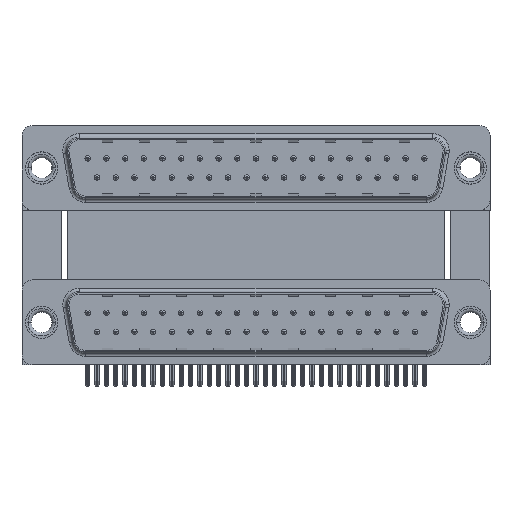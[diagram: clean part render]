
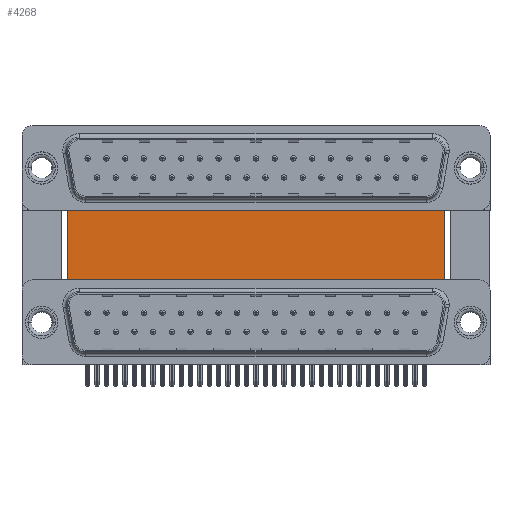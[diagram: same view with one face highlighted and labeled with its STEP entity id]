
A CAD part, top view. The second image highlights one B-rep face of the part: STEP entity #4268.
In plain terms, the highlighted planar face has unit normal (0, 0, 1).
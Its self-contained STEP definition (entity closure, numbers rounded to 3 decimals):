
#3031 = ORIENTED_EDGE ( 'NONE', *, *, #50765, .F. ) ;
#3351 = VECTOR ( 'NONE', #49245, 1000. ) ;
#4268 = ADVANCED_FACE ( 'NONE', ( #32159 ), #43980, .F. ) ;
#5175 = CARTESIAN_POINT ( 'NONE',  ( 3.79, 16.585, -12. ) ) ;
#9388 = CARTESIAN_POINT ( 'NONE',  ( 3.79, 16.585, -12. ) ) ;
#11183 = VECTOR ( 'NONE', #44764, 1000. ) ;
#13521 = CARTESIAN_POINT ( 'NONE',  ( 3.79, 16.585, -12. ) ) ;
#15374 = CARTESIAN_POINT ( 'NONE',  ( 59.71, -3.735, -12. ) ) ;
#17999 = VECTOR ( 'NONE', #21166, 1000. ) ;
#18813 = CARTESIAN_POINT ( 'NONE',  ( 59.71, 16.585, -12. ) ) ;
#19099 = VERTEX_POINT ( 'NONE', #15374 ) ;
#21166 = DIRECTION ( 'NONE',  ( 1., 0., 0. ) ) ;
#21532 = ORIENTED_EDGE ( 'NONE', *, *, #44427, .T. ) ;
#21940 = ORIENTED_EDGE ( 'NONE', *, *, #35504, .F. ) ;
#22211 = DIRECTION ( 'NONE',  ( 0., -1., 0. ) ) ;
#23934 = DIRECTION ( 'NONE',  ( 0., 0., -1. ) ) ;
#24720 = LINE ( 'NONE', #5175, #11183 ) ;
#26570 = LINE ( 'NONE', #42001, #46527 ) ;
#28113 = CARTESIAN_POINT ( 'NONE',  ( 3.79, -3.735, -12. ) ) ;
#28541 = DIRECTION ( 'NONE',  ( -1., 0., 0. ) ) ;
#32159 = FACE_OUTER_BOUND ( 'NONE', #48463, .T. ) ;
#32413 = CARTESIAN_POINT ( 'NONE',  ( 3.79, 16.585, -12. ) ) ;
#33258 = LINE ( 'NONE', #40709, #17999 ) ;
#33548 = LINE ( 'NONE', #9388, #3351 ) ;
#35504 = EDGE_CURVE ( 'NONE', #45365, #39340, #33548, .T. ) ;
#35865 = VERTEX_POINT ( 'NONE', #28113 ) ;
#39340 = VERTEX_POINT ( 'NONE', #18813 ) ;
#40136 = AXIS2_PLACEMENT_3D ( 'NONE', #32413, #23934, #28541 ) ;
#40709 = CARTESIAN_POINT ( 'NONE',  ( 3.79, -3.735, -12. ) ) ;
#40868 = ORIENTED_EDGE ( 'NONE', *, *, #48098, .T. ) ;
#42001 = CARTESIAN_POINT ( 'NONE',  ( 59.71, 16.585, -12. ) ) ;
#43980 = PLANE ( 'NONE',  #40136 ) ;
#44427 = EDGE_CURVE ( 'NONE', #45365, #35865, #24720, .T. ) ;
#44764 = DIRECTION ( 'NONE',  ( 0., -1., 0. ) ) ;
#45365 = VERTEX_POINT ( 'NONE', #13521 ) ;
#46527 = VECTOR ( 'NONE', #22211, 1000. ) ;
#48098 = EDGE_CURVE ( 'NONE', #35865, #19099, #33258, .T. ) ;
#48463 = EDGE_LOOP ( 'NONE', ( #40868, #3031, #21940, #21532 ) ) ;
#49245 = DIRECTION ( 'NONE',  ( 1., 0., 0. ) ) ;
#50765 = EDGE_CURVE ( 'NONE', #39340, #19099, #26570, .T. ) ;
